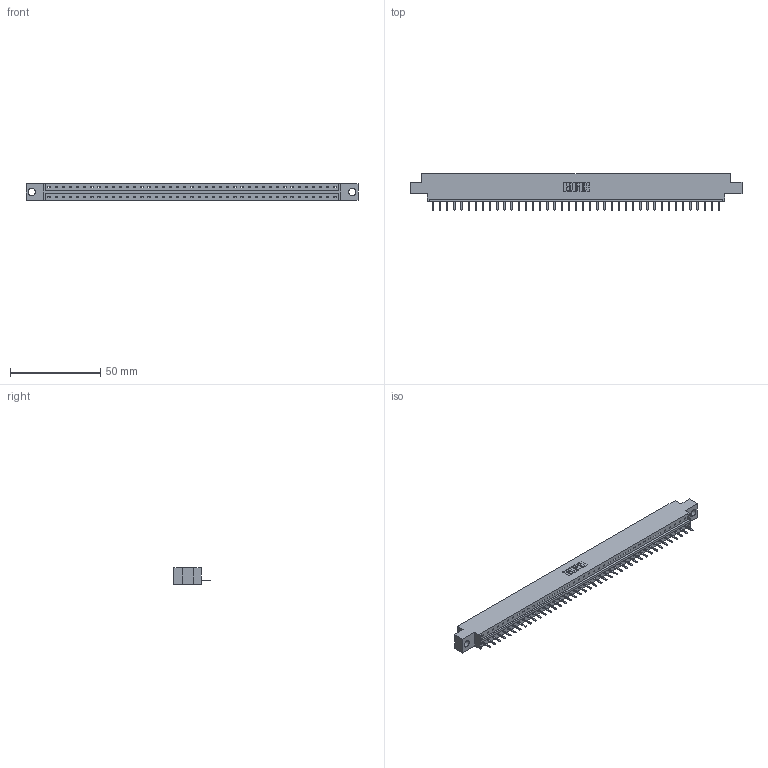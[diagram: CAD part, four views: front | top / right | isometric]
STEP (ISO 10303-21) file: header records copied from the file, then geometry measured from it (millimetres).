
FILE_DESCRIPTION (( 'STEP AP203' ), '1' );
FILE_NAME ('833-041-520-604.STEP', '2020-06-03T18:40:53', ( '' ), ( '' ), 'SwSTEP 2.0', 'SolidWorks 2020', '' );
FILE_SCHEMA (( 'CONFIG_CONTROL_DESIGN' ));
Length unit declared in the file: inch
Products named in the file (3): 833 Part_Offset - .156 Dia - TH; 345-292-001_345-293-120; 833-041-520-604
Assembly tree (42 placements, depth 2):
  833-041-520-604
    833 Part_Offset - .156 Dia - TH
    345-292-001_345-293-120  x41
Bounding box: 184 x 20.02 x 9.4 mm (x, y, z)
Volume: 18073.2 mm3; surface area: 19128 mm2
Topology: 42 solids, 42 shells, 2660 faces, 7867 edges, 5134 vertices
Faces by surface type: plane 1878, cylinder 782
Entity records: 25443 total; most frequent: CARTESIAN_POINT 4409, ORIENTED_EDGE 4374, DIRECTION 3709, EDGE_CURVE 2187, LINE 2055, VECTOR 2055, VERTEX_POINT 1454, AXIS2_PLACEMENT_3D 827
